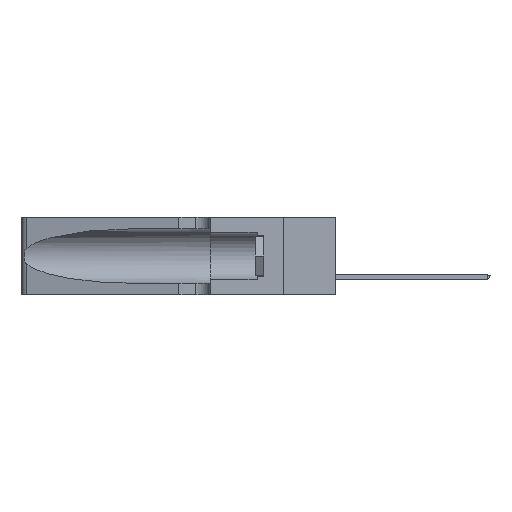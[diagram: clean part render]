
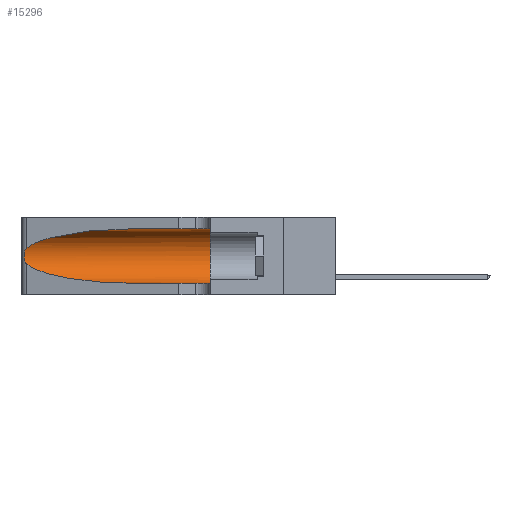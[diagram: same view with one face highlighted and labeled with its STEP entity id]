
A CAD part, left-side view. The second image highlights one B-rep face of the part: STEP entity #15296.
In plain terms, the highlighted cylindrical face has radius 3.308 mm (diameter 6.617 mm), a partial arc.
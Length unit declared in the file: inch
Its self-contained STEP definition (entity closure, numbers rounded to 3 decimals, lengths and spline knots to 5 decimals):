
#237 = CARTESIAN_POINT ( 'NONE',  ( 0.1305, 1.61858, 0.185 ) ) ;
#426 = CIRCLE ( 'NONE', #8650, 0.13025 ) ;
#868 = CARTESIAN_POINT ( 'NONE',  ( 0.25787, 1.23484, 0.2124 ) ) ;
#1133 = CARTESIAN_POINT ( 'NONE',  ( 0.25555, 1.22993, 0.14849 ) ) ;
#1205 = EDGE_CURVE ( 'NONE', #18337, #7298, #17097, .T. ) ;
#1673 = EDGE_LOOP ( 'NONE', ( #14765, #18102, #24071, #6165, #12668, #21948 ) ) ;
#2755 = VERTEX_POINT ( 'NONE', #20625 ) ;
#2899 = CARTESIAN_POINT ( 'NONE',  ( 0.26018, 1.23835, 0.19895 ) ) ;
#2905 = VECTOR ( 'NONE', #16074, 39.37008 ) ;
#3138 = CARTESIAN_POINT ( 'NONE',  ( 0.1305, 0.35, 0.05475 ) ) ;
#4330 = VERTEX_POINT ( 'NONE', #8847 ) ;
#4937 = CARTESIAN_POINT ( 'NONE',  ( 0.26075, 1.23896, 0.19203 ) ) ;
#5117 = CYLINDRICAL_SURFACE ( 'NONE', #25965, 0.13025 ) ;
#6165 = ORIENTED_EDGE ( 'NONE', *, *, #1205, .T. ) ;
#6536 = EDGE_CURVE ( 'NONE', #7498, #7298, #426, .T. ) ;
#6621 = VECTOR ( 'NONE', #18883, 39.37008 ) ;
#6930 = CARTESIAN_POINT ( 'NONE',  ( 0.25487, 1.22718, 0.14631 ) ) ;
#7298 = VERTEX_POINT ( 'NONE', #3138 ) ;
#7498 = VERTEX_POINT ( 'NONE', #25812 ) ;
#7608 = FACE_OUTER_BOUND ( 'NONE', #1673, .T. ) ;
#8572 = CARTESIAN_POINT ( 'NONE',  ( 0.25487, 1.22718, 0.22369 ) ) ;
#8650 = AXIS2_PLACEMENT_3D ( 'NONE', #23436, #17383, #13440 ) ;
#8793 = CARTESIAN_POINT ( 'NONE',  ( 0.25639, 1.23184, 0.21858 ) ) ;
#8847 = CARTESIAN_POINT ( 'NONE',  ( 0.25487, 1.22718, 0.22369 ) ) ;
#8962 = CARTESIAN_POINT ( 'NONE',  ( 0.25555, 1.22994, 0.2215 ) ) ;
#9053 = CARTESIAN_POINT ( 'NONE',  ( 0.26075, 1.23896, 0.178 ) ) ;
#9190 =( BOUNDED_CURVE ( )  B_SPLINE_CURVE ( 3, ( #21344, #13505, #21435, #15564 ),
 .UNSPECIFIED., .F., .F. ) 
 B_SPLINE_CURVE_WITH_KNOTS ( ( 4, 4 ),
 ( 3.44316, 4.71239 ),
 .UNSPECIFIED. ) 
 CURVE ( )  GEOMETRIC_REPRESENTATION_ITEM ( )  RATIONAL_B_SPLINE_CURVE ( ( 1., 0.87, 0.87, 1. ) ) 
 REPRESENTATION_ITEM ( '' )  );
#10408 = EDGE_CURVE ( 'NONE', #4330, #14620, #11585, .T. ) ;
#11585 = B_SPLINE_CURVE_WITH_KNOTS ( 'NONE', 3,
 ( #21084, #8962, #8793, #868, #23148, #2899, #4937, #9053, #19139, #25213, #19051, #25120, #1133, #6930 ),
 .UNSPECIFIED., .F., .F.,
 ( 4, 2, 2, 2, 2, 2, 4 ),
 ( 0., 0.00027, 0.00053, 0.00107, 0.0016, 0.00187, 0.00214 ),
 .UNSPECIFIED. ) ;
#12355 =( BOUNDED_CURVE ( )  B_SPLINE_CURVE ( 3, ( #24405, #14475, #16336, #8572 ),
 .UNSPECIFIED., .F., .T. ) 
 B_SPLINE_CURVE_WITH_KNOTS ( ( 4, 4 ),
 ( 1.5708, 2.84003 ),
 .UNSPECIFIED. ) 
 CURVE ( )  GEOMETRIC_REPRESENTATION_ITEM ( )  RATIONAL_B_SPLINE_CURVE ( ( 1., 0.87, 0.87, 1. ) ) 
 REPRESENTATION_ITEM ( '' )  );
#12668 = ORIENTED_EDGE ( 'NONE', *, *, #6536, .F. ) ;
#13440 = DIRECTION ( 'NONE',  ( 0., 0., 1. ) ) ;
#13505 = CARTESIAN_POINT ( 'NONE',  ( 0.2373, 1.15595, 0.08982 ) ) ;
#14178 = LINE ( 'NONE', #17106, #6621 ) ;
#14475 = CARTESIAN_POINT ( 'NONE',  ( 0.18966, 0.96281, 0.31525 ) ) ;
#14531 = DIRECTION ( 'NONE',  ( 0., -1., 0. ) ) ;
#14620 = VERTEX_POINT ( 'NONE', #22212 ) ;
#14765 = ORIENTED_EDGE ( 'NONE', *, *, #18929, .T. ) ;
#14800 = CARTESIAN_POINT ( 'NONE',  ( 0.1305, 0.72297, 0.05475 ) ) ;
#14806 = DIRECTION ( 'NONE',  ( 0., 0., -1. ) ) ;
#15296 = ADVANCED_FACE ( 'NONE', ( #7608 ), #5117, .F. ) ;
#15564 = CARTESIAN_POINT ( 'NONE',  ( 0.1305, 0.72297, 0.05475 ) ) ;
#16074 = DIRECTION ( 'NONE',  ( 0., -1., 0. ) ) ;
#16336 = CARTESIAN_POINT ( 'NONE',  ( 0.2373, 1.15595, 0.28018 ) ) ;
#17097 = LINE ( 'NONE', #20086, #2905 ) ;
#17106 = CARTESIAN_POINT ( 'NONE',  ( 0.1305, 1.61858, 0.31525 ) ) ;
#17383 = DIRECTION ( 'NONE',  ( 0., 1., 0. ) ) ;
#18102 = ORIENTED_EDGE ( 'NONE', *, *, #10408, .T. ) ;
#18337 = VERTEX_POINT ( 'NONE', #14800 ) ;
#18883 = DIRECTION ( 'NONE',  ( 0., -1., 0. ) ) ;
#18929 = EDGE_CURVE ( 'NONE', #2755, #4330, #12355, .T. ) ;
#19051 = CARTESIAN_POINT ( 'NONE',  ( 0.25789, 1.23486, 0.15765 ) ) ;
#19139 = CARTESIAN_POINT ( 'NONE',  ( 0.26017, 1.23833, 0.17102 ) ) ;
#20086 = CARTESIAN_POINT ( 'NONE',  ( 0.1305, 1.61858, 0.05475 ) ) ;
#20579 = EDGE_CURVE ( 'NONE', #14620, #18337, #9190, .T. ) ;
#20625 = CARTESIAN_POINT ( 'NONE',  ( 0.1305, 0.72297, 0.31525 ) ) ;
#21084 = CARTESIAN_POINT ( 'NONE',  ( 0.25487, 1.22718, 0.22369 ) ) ;
#21344 = CARTESIAN_POINT ( 'NONE',  ( 0.25487, 1.22718, 0.14631 ) ) ;
#21435 = CARTESIAN_POINT ( 'NONE',  ( 0.18966, 0.96281, 0.05475 ) ) ;
#21948 = ORIENTED_EDGE ( 'NONE', *, *, #25971, .F. ) ;
#22212 = CARTESIAN_POINT ( 'NONE',  ( 0.25487, 1.22718, 0.14631 ) ) ;
#23148 = CARTESIAN_POINT ( 'NONE',  ( 0.25854, 1.2359, 0.20912 ) ) ;
#23436 = CARTESIAN_POINT ( 'NONE',  ( 0.1305, 0.35, 0.185 ) ) ;
#24071 = ORIENTED_EDGE ( 'NONE', *, *, #20579, .T. ) ;
#24405 = CARTESIAN_POINT ( 'NONE',  ( 0.1305, 0.72297, 0.31525 ) ) ;
#25120 = CARTESIAN_POINT ( 'NONE',  ( 0.25639, 1.23186, 0.15144 ) ) ;
#25213 = CARTESIAN_POINT ( 'NONE',  ( 0.25856, 1.23593, 0.16098 ) ) ;
#25812 = CARTESIAN_POINT ( 'NONE',  ( 0.1305, 0.35, 0.31525 ) ) ;
#25965 = AXIS2_PLACEMENT_3D ( 'NONE', #237, #14531, #14806 ) ;
#25971 = EDGE_CURVE ( 'NONE', #2755, #7498, #14178, .T. ) ;
